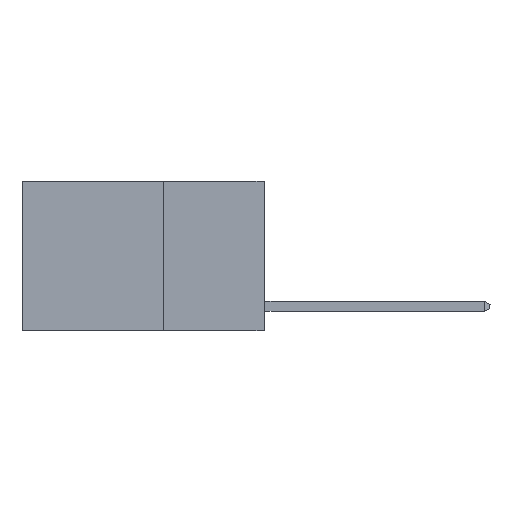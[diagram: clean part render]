
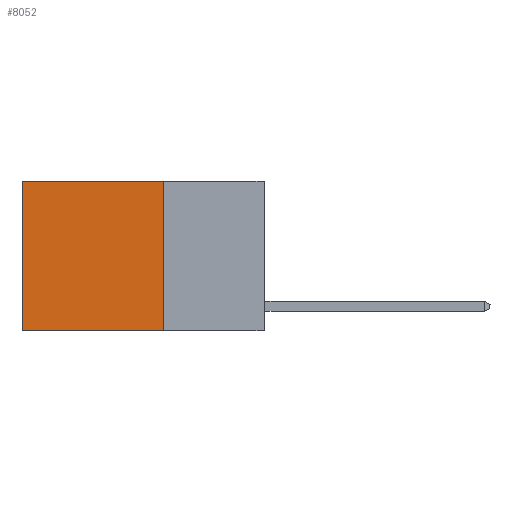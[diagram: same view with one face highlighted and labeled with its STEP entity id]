
A CAD part, left-side view. The second image highlights one B-rep face of the part: STEP entity #8052.
In plain terms, the highlighted planar face has unit normal (-1, 0, 0).
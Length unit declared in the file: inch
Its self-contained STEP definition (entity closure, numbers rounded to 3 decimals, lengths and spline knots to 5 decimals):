
#913 = DIRECTION ( 'NONE',  ( 1., 0., 0. ) ) ;
#921 = VECTOR ( 'NONE', #2238, 39.37008 ) ;
#1176 = CARTESIAN_POINT ( 'NONE',  ( 0.2625, 0.25, -0.37 ) ) ;
#2238 = DIRECTION ( 'NONE',  ( 0., 1., 0. ) ) ;
#2435 = CARTESIAN_POINT ( 'NONE',  ( 0.2625, 0.6, 0. ) ) ;
#3115 = ORIENTED_EDGE ( 'NONE', *, *, #5749, .T. ) ;
#3330 = VERTEX_POINT ( 'NONE', #9412 ) ;
#3495 = VERTEX_POINT ( 'NONE', #9769 ) ;
#3653 = LINE ( 'NONE', #1176, #921 ) ;
#3764 = DIRECTION ( 'NONE',  ( 0., 0., -1. ) ) ;
#4163 = LINE ( 'NONE', #10336, #12472 ) ;
#4257 = VECTOR ( 'NONE', #3764, 39.37008 ) ;
#5530 = ORIENTED_EDGE ( 'NONE', *, *, #11216, .F. ) ;
#5749 = EDGE_CURVE ( 'NONE', #3495, #6142, #5871, .T. ) ;
#5871 = LINE ( 'NONE', #2435, #11127 ) ;
#5884 = EDGE_CURVE ( 'NONE', #12517, #3330, #9488, .T. ) ;
#6042 = PLANE ( 'NONE',  #6210 ) ;
#6142 = VERTEX_POINT ( 'NONE', #7301 ) ;
#6210 = AXIS2_PLACEMENT_3D ( 'NONE', #7110, #913, #8167 ) ;
#7110 = CARTESIAN_POINT ( 'NONE',  ( 0.2625, 0.25, 0. ) ) ;
#7301 = CARTESIAN_POINT ( 'NONE',  ( 0.2625, 0.6, -0.37 ) ) ;
#7618 = CARTESIAN_POINT ( 'NONE',  ( 0.2625, 0.25, 0. ) ) ;
#8052 = ADVANCED_FACE ( 'NONE', ( #12372 ), #6042, .F. ) ;
#8167 = DIRECTION ( 'NONE',  ( 0., 0., -1. ) ) ;
#9284 = DIRECTION ( 'NONE',  ( 0., 1., 0. ) ) ;
#9412 = CARTESIAN_POINT ( 'NONE',  ( 0.2625, 0.25, -0.37 ) ) ;
#9488 = LINE ( 'NONE', #13121, #4257 ) ;
#9751 = ORIENTED_EDGE ( 'NONE', *, *, #10515, .T. ) ;
#9769 = CARTESIAN_POINT ( 'NONE',  ( 0.2625, 0.6, 0. ) ) ;
#10336 = CARTESIAN_POINT ( 'NONE',  ( 0.2625, 0.25, 0. ) ) ;
#10515 = EDGE_CURVE ( 'NONE', #12517, #3495, #4163, .T. ) ;
#11127 = VECTOR ( 'NONE', #12888, 39.37008 ) ;
#11216 = EDGE_CURVE ( 'NONE', #3330, #6142, #3653, .T. ) ;
#11339 = ORIENTED_EDGE ( 'NONE', *, *, #5884, .F. ) ;
#11390 = EDGE_LOOP ( 'NONE', ( #3115, #5530, #11339, #9751 ) ) ;
#12372 = FACE_OUTER_BOUND ( 'NONE', #11390, .T. ) ;
#12472 = VECTOR ( 'NONE', #9284, 39.37008 ) ;
#12517 = VERTEX_POINT ( 'NONE', #7618 ) ;
#12888 = DIRECTION ( 'NONE',  ( 0., 0., -1. ) ) ;
#13121 = CARTESIAN_POINT ( 'NONE',  ( 0.2625, 0.25, 0. ) ) ;
